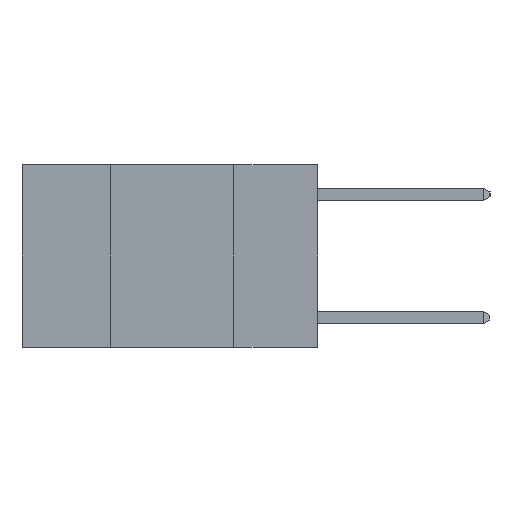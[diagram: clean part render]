
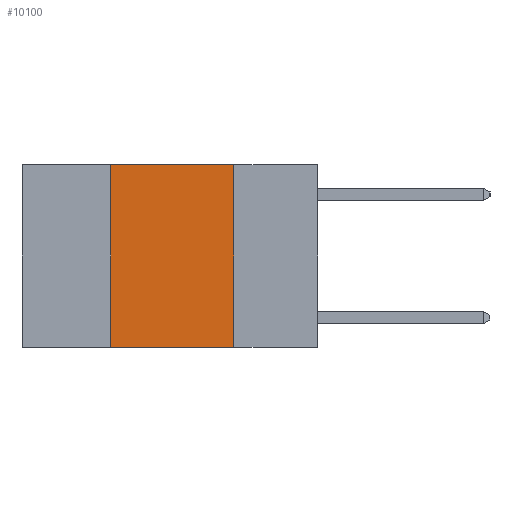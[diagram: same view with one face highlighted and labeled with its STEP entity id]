
A CAD part, left-side view. The second image highlights one B-rep face of the part: STEP entity #10100.
In plain terms, the highlighted planar face has unit normal (-1, 0, 0).
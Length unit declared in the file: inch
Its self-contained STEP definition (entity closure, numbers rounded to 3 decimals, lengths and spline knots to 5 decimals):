
#138 = DIRECTION ( 'NONE',  ( 0., -1., 0. ) ) ;
#161 = ORIENTED_EDGE ( 'NONE', *, *, #6348, .F. ) ;
#196 = ORIENTED_EDGE ( 'NONE', *, *, #7069, .F. ) ;
#254 = ORIENTED_EDGE ( 'NONE', *, *, #4152, .F. ) ;
#266 = ORIENTED_EDGE ( 'NONE', *, *, #9298, .T. ) ;
#428 = LINE ( 'NONE', #8862, #2854 ) ;
#817 = LINE ( 'NONE', #6094, #6367 ) ;
#825 = VECTOR ( 'NONE', #5758, 39.37008 ) ;
#845 = CARTESIAN_POINT ( 'NONE',  ( 0., 0.6, 0. ) ) ;
#1013 = LINE ( 'NONE', #11192, #5957 ) ;
#1198 = EDGE_LOOP ( 'NONE', ( #161, #196, #254, #266 ) ) ;
#1405 = CARTESIAN_POINT ( 'NONE',  ( 0., 0.42, 0. ) ) ;
#1909 = DIRECTION ( 'NONE',  ( 0., 0., -1. ) ) ;
#1991 = VERTEX_POINT ( 'NONE', #3204 ) ;
#2436 = FACE_OUTER_BOUND ( 'NONE', #1198, .T. ) ;
#2504 = VERTEX_POINT ( 'NONE', #7050 ) ;
#2854 = VECTOR ( 'NONE', #3237, 39.37008 ) ;
#3204 = CARTESIAN_POINT ( 'NONE',  ( 0., 0.17, 0. ) ) ;
#3237 = DIRECTION ( 'NONE',  ( 0., 0., 1. ) ) ;
#4152 = EDGE_CURVE ( 'NONE', #5279, #11788, #428, .T. ) ;
#5279 = VERTEX_POINT ( 'NONE', #5798 ) ;
#5688 = DIRECTION ( 'NONE',  ( 0., 0., -1. ) ) ;
#5758 = DIRECTION ( 'NONE',  ( 0., -1., 0. ) ) ;
#5798 = CARTESIAN_POINT ( 'NONE',  ( 0., 0.42, -0.37 ) ) ;
#5957 = VECTOR ( 'NONE', #5688, 39.37008 ) ;
#6094 = CARTESIAN_POINT ( 'NONE',  ( 0., 0.6, -0.37 ) ) ;
#6348 = EDGE_CURVE ( 'NONE', #1991, #2504, #1013, .T. ) ;
#6367 = VECTOR ( 'NONE', #138, 39.37008 ) ;
#7050 = CARTESIAN_POINT ( 'NONE',  ( 0., 0.17, -0.37 ) ) ;
#7069 = EDGE_CURVE ( 'NONE', #11788, #1991, #10966, .T. ) ;
#7637 = DIRECTION ( 'NONE',  ( 1., 0., 0. ) ) ;
#8862 = CARTESIAN_POINT ( 'NONE',  ( 0., 0.42, 0. ) ) ;
#9298 = EDGE_CURVE ( 'NONE', #5279, #2504, #817, .T. ) ;
#10100 = ADVANCED_FACE ( 'NONE', ( #2436 ), #11283, .F. ) ;
#10966 = LINE ( 'NONE', #12218, #825 ) ;
#11192 = CARTESIAN_POINT ( 'NONE',  ( 0., 0.17, 0. ) ) ;
#11283 = PLANE ( 'NONE',  #12081 ) ;
#11788 = VERTEX_POINT ( 'NONE', #1405 ) ;
#12081 = AXIS2_PLACEMENT_3D ( 'NONE', #845, #7637, #1909 ) ;
#12218 = CARTESIAN_POINT ( 'NONE',  ( 0., 0.6, 0. ) ) ;
